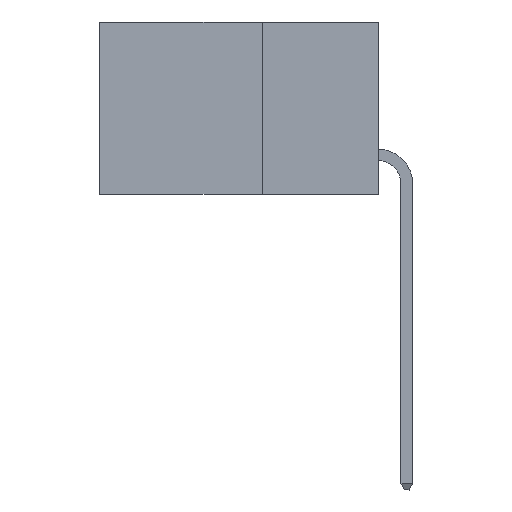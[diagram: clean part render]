
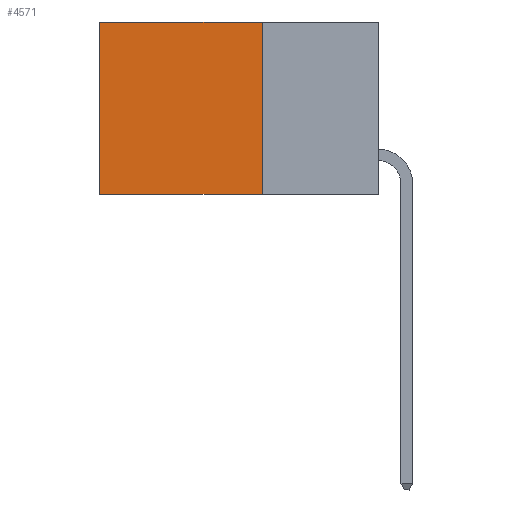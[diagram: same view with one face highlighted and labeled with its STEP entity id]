
A CAD part, left-side view. The second image highlights one B-rep face of the part: STEP entity #4571.
In plain terms, the highlighted planar face has unit normal (-1, 0, 0).
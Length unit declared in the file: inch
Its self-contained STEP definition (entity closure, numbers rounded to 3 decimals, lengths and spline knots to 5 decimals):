
#91 = ORIENTED_EDGE ( 'NONE', *, *, #2153, .T. ) ;
#1106 = CARTESIAN_POINT ( 'NONE',  ( 0.2615, 0.6, -0.37 ) ) ;
#1182 = DIRECTION ( 'NONE',  ( 0., 1., 0. ) ) ;
#1330 = LINE ( 'NONE', #3436, #9412 ) ;
#1583 = EDGE_CURVE ( 'NONE', #7119, #7217, #1330, .T. ) ;
#2080 = AXIS2_PLACEMENT_3D ( 'NONE', #10010, #7812, #12060 ) ;
#2153 = EDGE_CURVE ( 'NONE', #5845, #7083, #13057, .T. ) ;
#2397 = FACE_OUTER_BOUND ( 'NONE', #10291, .T. ) ;
#3186 = DIRECTION ( 'NONE',  ( 0., 0., -1. ) ) ;
#3436 = CARTESIAN_POINT ( 'NONE',  ( 0.2615, 0.25, -0.37 ) ) ;
#4571 = ADVANCED_FACE ( 'NONE', ( #2397 ), #7738, .F. ) ;
#4754 = VECTOR ( 'NONE', #1182, 39.37008 ) ;
#5845 = VERTEX_POINT ( 'NONE', #10931 ) ;
#6472 = VECTOR ( 'NONE', #3186, 39.37008 ) ;
#7049 = ORIENTED_EDGE ( 'NONE', *, *, #10119, .T. ) ;
#7083 = VERTEX_POINT ( 'NONE', #8141 ) ;
#7119 = VERTEX_POINT ( 'NONE', #9143 ) ;
#7217 = VERTEX_POINT ( 'NONE', #1106 ) ;
#7438 = ORIENTED_EDGE ( 'NONE', *, *, #1583, .F. ) ;
#7631 = LINE ( 'NONE', #9616, #6472 ) ;
#7738 = PLANE ( 'NONE',  #2080 ) ;
#7812 = DIRECTION ( 'NONE',  ( 1., 0., 0. ) ) ;
#7942 = VECTOR ( 'NONE', #10279, 39.37008 ) ;
#8141 = CARTESIAN_POINT ( 'NONE',  ( 0.2615, 0.6, 0. ) ) ;
#8653 = CARTESIAN_POINT ( 'NONE',  ( 0.2615, 0.25, 0. ) ) ;
#8937 = DIRECTION ( 'NONE',  ( 0., 1., 0. ) ) ;
#9143 = CARTESIAN_POINT ( 'NONE',  ( 0.2615, 0.25, -0.37 ) ) ;
#9412 = VECTOR ( 'NONE', #8937, 39.37008 ) ;
#9414 = ORIENTED_EDGE ( 'NONE', *, *, #12666, .F. ) ;
#9616 = CARTESIAN_POINT ( 'NONE',  ( 0.2615, 0.6, -0.37 ) ) ;
#10010 = CARTESIAN_POINT ( 'NONE',  ( 0.2615, 0.25, -0.37 ) ) ;
#10119 = EDGE_CURVE ( 'NONE', #7083, #7217, #7631, .T. ) ;
#10279 = DIRECTION ( 'NONE',  ( 0., 0., -1. ) ) ;
#10291 = EDGE_LOOP ( 'NONE', ( #7049, #7438, #9414, #91 ) ) ;
#10406 = LINE ( 'NONE', #11461, #7942 ) ;
#10931 = CARTESIAN_POINT ( 'NONE',  ( 0.2615, 0.25, 0. ) ) ;
#11461 = CARTESIAN_POINT ( 'NONE',  ( 0.2615, 0.25, -0.37 ) ) ;
#12060 = DIRECTION ( 'NONE',  ( 0., 0., -1. ) ) ;
#12666 = EDGE_CURVE ( 'NONE', #5845, #7119, #10406, .T. ) ;
#13057 = LINE ( 'NONE', #8653, #4754 ) ;
